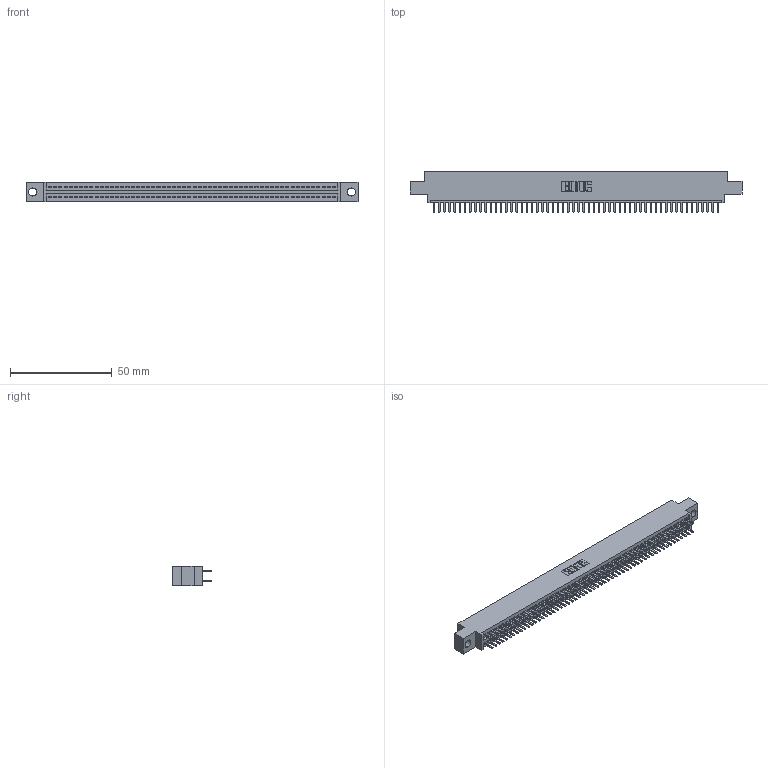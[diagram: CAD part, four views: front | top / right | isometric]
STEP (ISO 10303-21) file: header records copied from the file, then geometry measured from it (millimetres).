
FILE_DESCRIPTION (( 'STEP AP203' ), '1' );
FILE_NAME ('345-112-520-804.STEP', '2018-10-07T13:41:31', ( '' ), ( '' ), 'SwSTEP 2.0', 'SolidWorks 2016', '' );
FILE_SCHEMA (( 'CONFIG_CONTROL_DESIGN' ));
Length unit declared in the file: inch
Products named in the file (3): 345 Part_0.170 Offset - 0.156 Dia-TH; 345-112-520-804; 345-292-001_345-293-120
Assembly tree (113 placements, depth 2):
  345-112-520-804
    345 Part_0.170 Offset - 0.156 Dia-TH
    345-292-001_345-293-120  x112
Bounding box: 163.45 x 19.68 x 9.4 mm (x, y, z)
Volume: 15757.1 mm3; surface area: 23416.7 mm2
Topology: 113 solids, 113 shells, 6178 faces, 17937 edges, 11658 vertices
Faces by surface type: plane 4004, cylinder 2174
Entity records: 42303 total; most frequent: CARTESIAN_POINT 7092, ORIENTED_EDGE 7014, DIRECTION 6223, EDGE_CURVE 3507, VECTOR 3147, LINE 3147, VERTEX_POINT 2334, AXIS2_PLACEMENT_3D 1538
